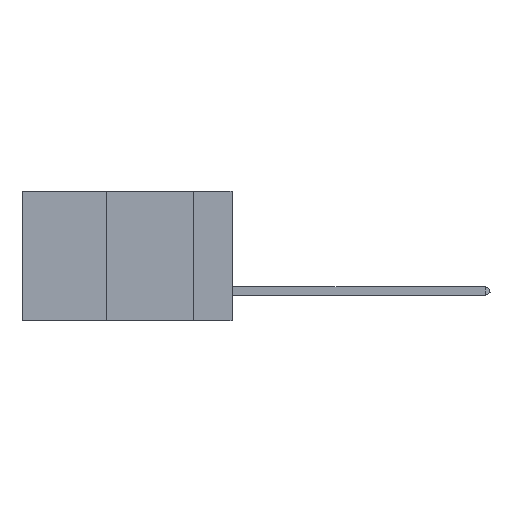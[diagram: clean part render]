
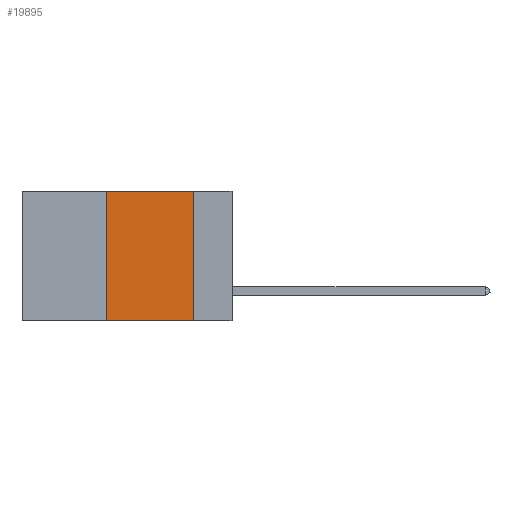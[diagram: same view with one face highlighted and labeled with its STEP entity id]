
A CAD part, left-side view. The second image highlights one B-rep face of the part: STEP entity #19895.
In plain terms, the highlighted planar face has unit normal (-1, 0, 0).
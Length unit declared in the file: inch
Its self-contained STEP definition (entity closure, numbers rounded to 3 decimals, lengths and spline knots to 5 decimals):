
#268 = CARTESIAN_POINT ( 'NONE',  ( 0., 0.11, 0. ) ) ;
#560 = LINE ( 'NONE', #27028, #21814 ) ;
#1609 = FACE_OUTER_BOUND ( 'NONE', #7711, .T. ) ;
#1936 = AXIS2_PLACEMENT_3D ( 'NONE', #28215, #17201, #25513 ) ;
#4523 = EDGE_CURVE ( 'NONE', #26944, #20437, #22271, .T. ) ;
#5903 = EDGE_CURVE ( 'NONE', #23621, #26944, #560, .T. ) ;
#7578 = VERTEX_POINT ( 'NONE', #12061 ) ;
#7711 = EDGE_LOOP ( 'NONE', ( #22540, #15273, #9646, #8981 ) ) ;
#7956 = CARTESIAN_POINT ( 'NONE',  ( 0., 0.36, 0. ) ) ;
#8981 = ORIENTED_EDGE ( 'NONE', *, *, #21504, .T. ) ;
#9286 = DIRECTION ( 'NONE',  ( 0., -1., 0. ) ) ;
#9646 = ORIENTED_EDGE ( 'NONE', *, *, #24433, .F. ) ;
#9834 = VECTOR ( 'NONE', #18347, 39.37008 ) ;
#12061 = CARTESIAN_POINT ( 'NONE',  ( 0., 0.36, -0.37 ) ) ;
#13159 = DIRECTION ( 'NONE',  ( 0., -1., 0. ) ) ;
#14577 = CARTESIAN_POINT ( 'NONE',  ( 0., 0.11, -0.37 ) ) ;
#15273 = ORIENTED_EDGE ( 'NONE', *, *, #5903, .F. ) ;
#15313 = CARTESIAN_POINT ( 'NONE',  ( 0., 0.6, -0.37 ) ) ;
#16480 = LINE ( 'NONE', #20784, #9834 ) ;
#17201 = DIRECTION ( 'NONE',  ( 1., 0., 0. ) ) ;
#18116 = CARTESIAN_POINT ( 'NONE',  ( 0., 0.11, 0. ) ) ;
#18347 = DIRECTION ( 'NONE',  ( 0., 0., 1. ) ) ;
#19895 = ADVANCED_FACE ( 'NONE', ( #1609 ), #23235, .F. ) ;
#20437 = VERTEX_POINT ( 'NONE', #14577 ) ;
#20784 = CARTESIAN_POINT ( 'NONE',  ( 0., 0.36, 0. ) ) ;
#21504 = EDGE_CURVE ( 'NONE', #7578, #20437, #24191, .T. ) ;
#21814 = VECTOR ( 'NONE', #9286, 39.37008 ) ;
#22271 = LINE ( 'NONE', #18116, #26063 ) ;
#22540 = ORIENTED_EDGE ( 'NONE', *, *, #4523, .F. ) ;
#22693 = DIRECTION ( 'NONE',  ( 0., 0., -1. ) ) ;
#23235 = PLANE ( 'NONE',  #1936 ) ;
#23621 = VERTEX_POINT ( 'NONE', #7956 ) ;
#24191 = LINE ( 'NONE', #15313, #27159 ) ;
#24433 = EDGE_CURVE ( 'NONE', #7578, #23621, #16480, .T. ) ;
#25513 = DIRECTION ( 'NONE',  ( 0., 0., -1. ) ) ;
#26063 = VECTOR ( 'NONE', #22693, 39.37008 ) ;
#26944 = VERTEX_POINT ( 'NONE', #268 ) ;
#27028 = CARTESIAN_POINT ( 'NONE',  ( 0., 0.6, 0. ) ) ;
#27159 = VECTOR ( 'NONE', #13159, 39.37008 ) ;
#28215 = CARTESIAN_POINT ( 'NONE',  ( 0., 0.6, 0. ) ) ;
